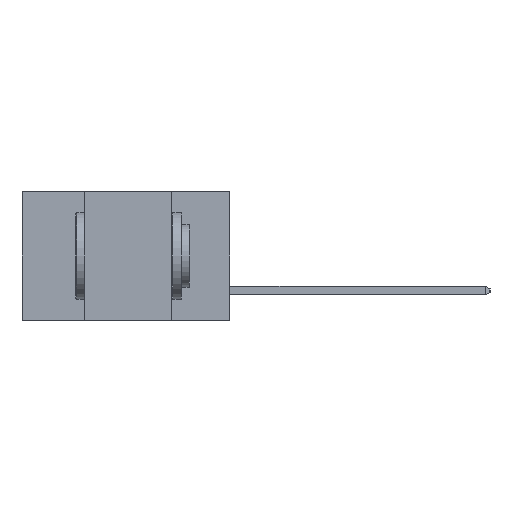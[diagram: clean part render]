
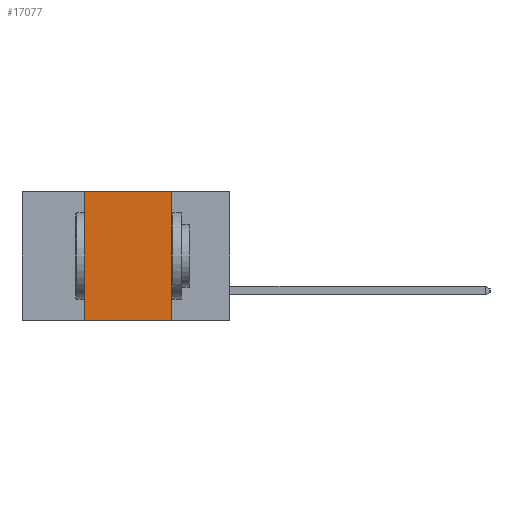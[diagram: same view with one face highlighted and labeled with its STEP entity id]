
A CAD part, left-side view. The second image highlights one B-rep face of the part: STEP entity #17077.
In plain terms, the highlighted planar face has unit normal (-1, 0, 0).
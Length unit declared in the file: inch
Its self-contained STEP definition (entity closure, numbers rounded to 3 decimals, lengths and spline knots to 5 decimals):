
#686 = VERTEX_POINT ( 'NONE', #8113 ) ;
#1686 = LINE ( 'NONE', #6039, #20563 ) ;
#2506 = VERTEX_POINT ( 'NONE', #18667 ) ;
#2576 = VECTOR ( 'NONE', #8640, 39.37008 ) ;
#2853 = VECTOR ( 'NONE', #19969, 39.37008 ) ;
#3203 = VERTEX_POINT ( 'NONE', #9826 ) ;
#3464 = EDGE_CURVE ( 'NONE', #686, #3203, #1686, .T. ) ;
#3469 = LINE ( 'NONE', #10925, #2853 ) ;
#4966 = PLANE ( 'NONE',  #12006 ) ;
#6039 = CARTESIAN_POINT ( 'NONE',  ( 0., 0.42, -0.37 ) ) ;
#6098 = DIRECTION ( 'NONE',  ( 0., 0., 1. ) ) ;
#6816 = DIRECTION ( 'NONE',  ( 1., 0., 0. ) ) ;
#7187 = VECTOR ( 'NONE', #13840, 39.37008 ) ;
#7440 = FACE_OUTER_BOUND ( 'NONE', #9366, .T. ) ;
#7514 = LINE ( 'NONE', #10499, #2576 ) ;
#8113 = CARTESIAN_POINT ( 'NONE',  ( 0., 0.42, -0.37 ) ) ;
#8640 = DIRECTION ( 'NONE',  ( 0., -1., 0. ) ) ;
#9366 = EDGE_LOOP ( 'NONE', ( #13486, #21273, #20209, #22577 ) ) ;
#9826 = CARTESIAN_POINT ( 'NONE',  ( 0., 0.42, 0. ) ) ;
#10499 = CARTESIAN_POINT ( 'NONE',  ( 0., 0.6, 0. ) ) ;
#10925 = CARTESIAN_POINT ( 'NONE',  ( 0., 0.17, -0.37 ) ) ;
#11287 = EDGE_CURVE ( 'NONE', #686, #12694, #17062, .T. ) ;
#12006 = AXIS2_PLACEMENT_3D ( 'NONE', #17899, #6816, #19621 ) ;
#12694 = VERTEX_POINT ( 'NONE', #18961 ) ;
#13486 = ORIENTED_EDGE ( 'NONE', *, *, #15932, .F. ) ;
#13840 = DIRECTION ( 'NONE',  ( 0., -1., 0. ) ) ;
#14444 = CARTESIAN_POINT ( 'NONE',  ( 0., 0.6, -0.37 ) ) ;
#15932 = EDGE_CURVE ( 'NONE', #2506, #12694, #3469, .T. ) ;
#17062 = LINE ( 'NONE', #14444, #7187 ) ;
#17077 = ADVANCED_FACE ( 'NONE', ( #7440 ), #4966, .F. ) ;
#17899 = CARTESIAN_POINT ( 'NONE',  ( 0., 0.6, 0. ) ) ;
#18667 = CARTESIAN_POINT ( 'NONE',  ( 0., 0.17, 0. ) ) ;
#18745 = EDGE_CURVE ( 'NONE', #3203, #2506, #7514, .T. ) ;
#18961 = CARTESIAN_POINT ( 'NONE',  ( 0., 0.17, -0.37 ) ) ;
#19621 = DIRECTION ( 'NONE',  ( 0., 0., -1. ) ) ;
#19969 = DIRECTION ( 'NONE',  ( 0., 0., -1. ) ) ;
#20209 = ORIENTED_EDGE ( 'NONE', *, *, #3464, .F. ) ;
#20563 = VECTOR ( 'NONE', #6098, 39.37008 ) ;
#21273 = ORIENTED_EDGE ( 'NONE', *, *, #18745, .F. ) ;
#22577 = ORIENTED_EDGE ( 'NONE', *, *, #11287, .T. ) ;
